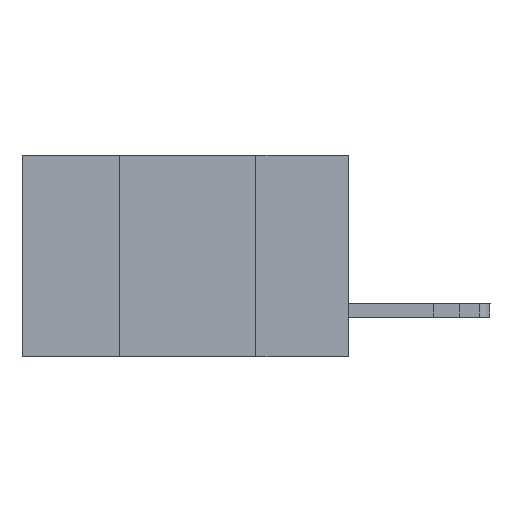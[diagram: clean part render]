
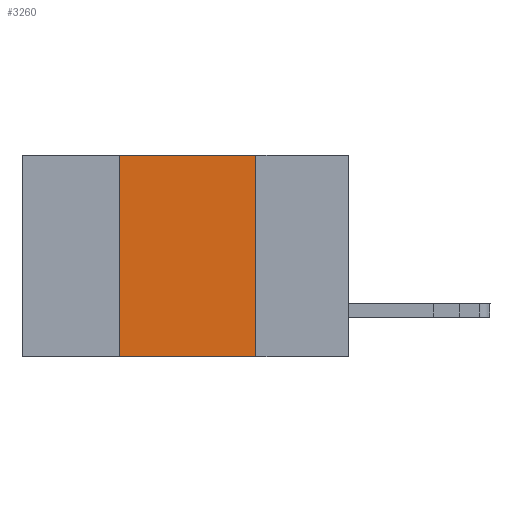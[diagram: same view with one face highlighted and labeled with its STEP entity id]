
A CAD part, left-side view. The second image highlights one B-rep face of the part: STEP entity #3260.
In plain terms, the highlighted planar face has unit normal (-1, 0, 0).
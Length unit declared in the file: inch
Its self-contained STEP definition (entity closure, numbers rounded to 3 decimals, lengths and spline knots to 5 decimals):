
#625 = ORIENTED_EDGE ( 'NONE', *, *, #6768, .F. ) ;
#686 = ORIENTED_EDGE ( 'NONE', *, *, #5010, .T. ) ;
#1198 = EDGE_CURVE ( 'NONE', #8864, #8515, #9748, .T. ) ;
#1389 = CARTESIAN_POINT ( 'NONE',  ( 0., 0.17, -0.37 ) ) ;
#1416 = VECTOR ( 'NONE', #8265, 39.37008 ) ;
#1624 = DIRECTION ( 'NONE',  ( 1., 0., 0. ) ) ;
#1681 = ORIENTED_EDGE ( 'NONE', *, *, #1198, .F. ) ;
#2547 = FACE_OUTER_BOUND ( 'NONE', #11002, .T. ) ;
#3260 = ADVANCED_FACE ( 'NONE', ( #2547 ), #6340, .F. ) ;
#3429 = EDGE_CURVE ( 'NONE', #8515, #5066, #8542, .T. ) ;
#4495 = DIRECTION ( 'NONE',  ( 0., 0., -1. ) ) ;
#4905 = VERTEX_POINT ( 'NONE', #12261 ) ;
#5010 = EDGE_CURVE ( 'NONE', #4905, #5066, #12194, .T. ) ;
#5066 = VERTEX_POINT ( 'NONE', #1389 ) ;
#6340 = PLANE ( 'NONE',  #8835 ) ;
#6768 = EDGE_CURVE ( 'NONE', #4905, #8864, #12041, .T. ) ;
#7487 = CARTESIAN_POINT ( 'NONE',  ( 0., 0.6, -0.37 ) ) ;
#7499 = DIRECTION ( 'NONE',  ( 0., 0., -1. ) ) ;
#7615 = CARTESIAN_POINT ( 'NONE',  ( 0., 0.17, -0.37 ) ) ;
#7855 = VECTOR ( 'NONE', #9806, 39.37008 ) ;
#8140 = CARTESIAN_POINT ( 'NONE',  ( 0., 0.42, 0. ) ) ;
#8246 = CARTESIAN_POINT ( 'NONE',  ( 0., 0.6, 0. ) ) ;
#8265 = DIRECTION ( 'NONE',  ( 0., 0., 1. ) ) ;
#8515 = VERTEX_POINT ( 'NONE', #10879 ) ;
#8542 = LINE ( 'NONE', #7615, #10258 ) ;
#8742 = VECTOR ( 'NONE', #11267, 39.37008 ) ;
#8835 = AXIS2_PLACEMENT_3D ( 'NONE', #8246, #1624, #4495 ) ;
#8864 = VERTEX_POINT ( 'NONE', #8140 ) ;
#9059 = CARTESIAN_POINT ( 'NONE',  ( 0., 0.42, -0.37 ) ) ;
#9748 = LINE ( 'NONE', #9919, #7855 ) ;
#9806 = DIRECTION ( 'NONE',  ( 0., -1., 0. ) ) ;
#9919 = CARTESIAN_POINT ( 'NONE',  ( 0., 0.6, 0. ) ) ;
#10192 = ORIENTED_EDGE ( 'NONE', *, *, #3429, .F. ) ;
#10258 = VECTOR ( 'NONE', #7499, 39.37008 ) ;
#10879 = CARTESIAN_POINT ( 'NONE',  ( 0., 0.17, 0. ) ) ;
#11002 = EDGE_LOOP ( 'NONE', ( #10192, #1681, #625, #686 ) ) ;
#11267 = DIRECTION ( 'NONE',  ( 0., -1., 0. ) ) ;
#12041 = LINE ( 'NONE', #9059, #1416 ) ;
#12194 = LINE ( 'NONE', #7487, #8742 ) ;
#12261 = CARTESIAN_POINT ( 'NONE',  ( 0., 0.42, -0.37 ) ) ;
